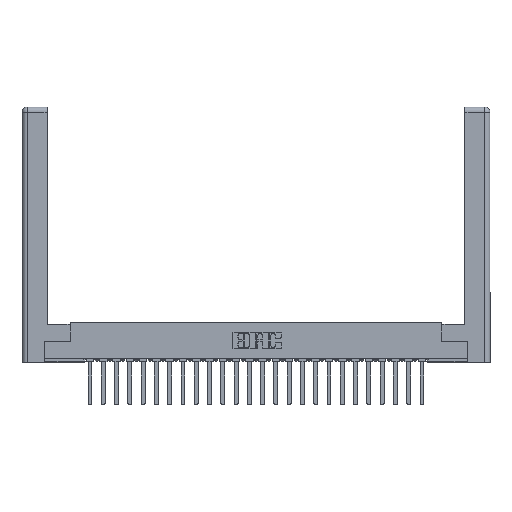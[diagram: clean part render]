
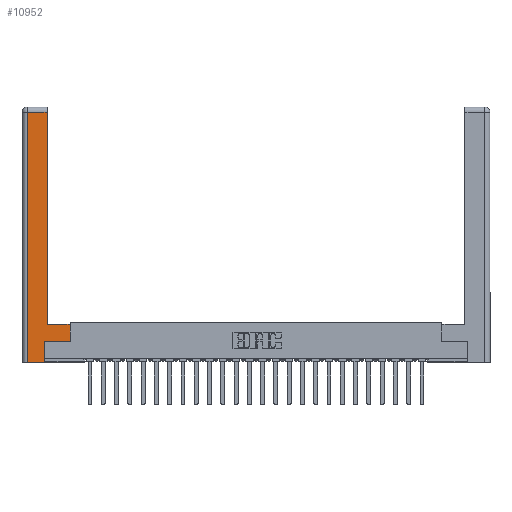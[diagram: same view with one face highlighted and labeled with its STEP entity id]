
A CAD part, top view. The second image highlights one B-rep face of the part: STEP entity #10952.
In plain terms, the highlighted planar face has unit normal (0, 0, 1).
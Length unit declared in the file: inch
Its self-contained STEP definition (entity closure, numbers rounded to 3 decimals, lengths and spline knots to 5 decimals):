
#289 = LINE ( 'NONE', #10510, #13096 ) ;
#711 = VECTOR ( 'NONE', #25403, 39.37008 ) ;
#824 = VECTOR ( 'NONE', #21490, 39.37008 ) ;
#966 = ORIENTED_EDGE ( 'NONE', *, *, #14378, .T. ) ;
#1109 = VERTEX_POINT ( 'NONE', #10914 ) ;
#2391 = CARTESIAN_POINT ( 'NONE',  ( 0.0615, 0., 0. ) ) ;
#2880 = VERTEX_POINT ( 'NONE', #3045 ) ;
#3045 = CARTESIAN_POINT ( 'NONE',  ( 0.565, 0.45, 0. ) ) ;
#3833 = CARTESIAN_POINT ( 'NONE',  ( 0.265, 0.245, 0. ) ) ;
#4741 = DIRECTION ( 'NONE',  ( 0., 1., 0. ) ) ;
#5273 = DIRECTION ( 'NONE',  ( -1., 0., 0. ) ) ;
#6685 = EDGE_CURVE ( 'NONE', #23920, #12663, #14376, .T. ) ;
#7006 = CARTESIAN_POINT ( 'NONE',  ( 0.265, 0., 0. ) ) ;
#7882 = VERTEX_POINT ( 'NONE', #10451 ) ;
#7896 = EDGE_CURVE ( 'NONE', #25196, #24962, #18986, .T. ) ;
#8305 = CARTESIAN_POINT ( 'NONE',  ( 0.0615, 2.94, 0. ) ) ;
#8553 = CARTESIAN_POINT ( 'NONE',  ( 0.0615, 0., 0. ) ) ;
#9510 = AXIS2_PLACEMENT_3D ( 'NONE', #20243, #18142, #5273 ) ;
#9742 = PLANE ( 'NONE',  #9510 ) ;
#9806 = VECTOR ( 'NONE', #4741, 39.37008 ) ;
#10021 = CARTESIAN_POINT ( 'NONE',  ( 0.265, 0., 0. ) ) ;
#10451 = CARTESIAN_POINT ( 'NONE',  ( 0.565, 0.245, 0. ) ) ;
#10510 = CARTESIAN_POINT ( 'NONE',  ( 0.295, 0.45, 0. ) ) ;
#10914 = CARTESIAN_POINT ( 'NONE',  ( 0.295, 0.45, 0. ) ) ;
#10952 = ADVANCED_FACE ( 'NONE', ( #13954 ), #9742, .F. ) ;
#11474 = VECTOR ( 'NONE', #23357, 39.37008 ) ;
#11867 = ORIENTED_EDGE ( 'NONE', *, *, #19056, .T. ) ;
#12663 = VERTEX_POINT ( 'NONE', #8305 ) ;
#13096 = VECTOR ( 'NONE', #19309, 39.37008 ) ;
#13449 = DIRECTION ( 'NONE',  ( 0., 1., 0. ) ) ;
#13954 = FACE_OUTER_BOUND ( 'NONE', #25213, .T. ) ;
#14376 = LINE ( 'NONE', #23016, #18258 ) ;
#14378 = EDGE_CURVE ( 'NONE', #12663, #20267, #25321, .T. ) ;
#14379 = ORIENTED_EDGE ( 'NONE', *, *, #22170, .T. ) ;
#15031 = ORIENTED_EDGE ( 'NONE', *, *, #25140, .T. ) ;
#15683 = CARTESIAN_POINT ( 'NONE',  ( 0.295, 3., 0. ) ) ;
#16117 = VECTOR ( 'NONE', #13449, 39.37008 ) ;
#17294 = LINE ( 'NONE', #25959, #824 ) ;
#17553 = EDGE_CURVE ( 'NONE', #24962, #7882, #17294, .T. ) ;
#18142 = DIRECTION ( 'NONE',  ( 0., 0., -1. ) ) ;
#18258 = VECTOR ( 'NONE', #22881, 39.37008 ) ;
#18560 = DIRECTION ( 'NONE',  ( 1., 0., 0. ) ) ;
#18986 = LINE ( 'NONE', #27505, #711 ) ;
#19056 = EDGE_CURVE ( 'NONE', #7882, #2880, #23886, .T. ) ;
#19309 = DIRECTION ( 'NONE',  ( -1., 0., 0. ) ) ;
#20118 = ORIENTED_EDGE ( 'NONE', *, *, #7896, .T. ) ;
#20243 = CARTESIAN_POINT ( 'NONE',  ( 0., 0., 0. ) ) ;
#20250 = CARTESIAN_POINT ( 'NONE',  ( 0.295, 2.94, 0. ) ) ;
#20267 = VERTEX_POINT ( 'NONE', #2391 ) ;
#20719 = ORIENTED_EDGE ( 'NONE', *, *, #26836, .T. ) ;
#21490 = DIRECTION ( 'NONE',  ( 1., 0., 0. ) ) ;
#21624 = ORIENTED_EDGE ( 'NONE', *, *, #6685, .T. ) ;
#21964 = LINE ( 'NONE', #15683, #16117 ) ;
#22170 = EDGE_CURVE ( 'NONE', #20267, #25196, #24976, .T. ) ;
#22737 = VECTOR ( 'NONE', #18560, 39.37008 ) ;
#22881 = DIRECTION ( 'NONE',  ( -1., 0., 0. ) ) ;
#23016 = CARTESIAN_POINT ( 'NONE',  ( 0.0615, 2.94, 0. ) ) ;
#23357 = DIRECTION ( 'NONE',  ( 0., -1., 0. ) ) ;
#23886 = LINE ( 'NONE', #26551, #9806 ) ;
#23920 = VERTEX_POINT ( 'NONE', #20250 ) ;
#24962 = VERTEX_POINT ( 'NONE', #3833 ) ;
#24976 = LINE ( 'NONE', #10021, #22737 ) ;
#25091 = ORIENTED_EDGE ( 'NONE', *, *, #17553, .T. ) ;
#25140 = EDGE_CURVE ( 'NONE', #1109, #23920, #21964, .T. ) ;
#25196 = VERTEX_POINT ( 'NONE', #7006 ) ;
#25213 = EDGE_LOOP ( 'NONE', ( #15031, #21624, #966, #14379, #20118, #25091, #11867, #20719 ) ) ;
#25321 = LINE ( 'NONE', #8553, #11474 ) ;
#25403 = DIRECTION ( 'NONE',  ( 0., 1., 0. ) ) ;
#25959 = CARTESIAN_POINT ( 'NONE',  ( 0.565, 0.245, 0. ) ) ;
#26551 = CARTESIAN_POINT ( 'NONE',  ( 0.565, 0.45, 0. ) ) ;
#26836 = EDGE_CURVE ( 'NONE', #2880, #1109, #289, .T. ) ;
#27505 = CARTESIAN_POINT ( 'NONE',  ( 0.265, 0.245, 0. ) ) ;
